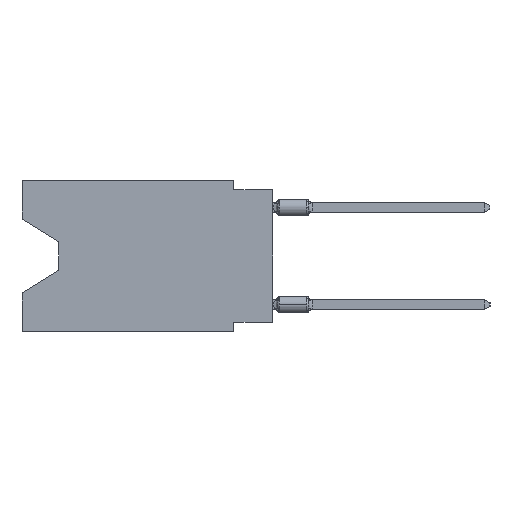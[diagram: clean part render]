
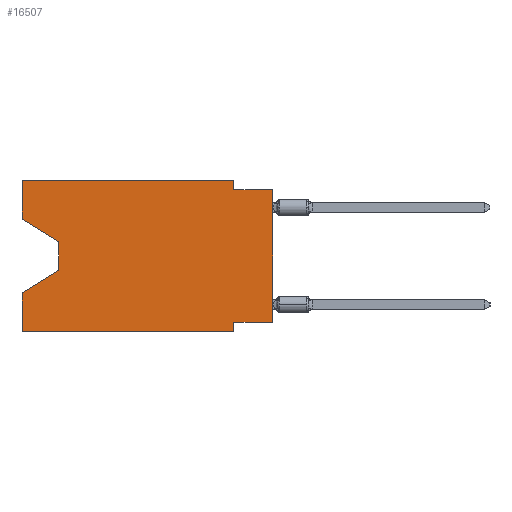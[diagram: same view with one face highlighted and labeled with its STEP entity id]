
A CAD part, left-side view. The second image highlights one B-rep face of the part: STEP entity #16507.
In plain terms, the highlighted planar face has unit normal (-1, 0, 0).
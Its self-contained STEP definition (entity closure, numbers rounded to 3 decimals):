
#143 = EDGE_CURVE ( 'NONE', #8141, #33290, #33464, .T. ) ;
#240 = CARTESIAN_POINT ( 'NONE',  ( 0., 16.383, 0. ) ) ;
#406 = ORIENTED_EDGE ( 'NONE', *, *, #2234, .F. ) ;
#1386 = DIRECTION ( 'NONE',  ( 0., 0.855, -0.519 ) ) ;
#1780 = EDGE_CURVE ( 'NONE', #19419, #35402, #20577, .T. ) ;
#2004 = CARTESIAN_POINT ( 'NONE',  ( 0., 16.383, 0. ) ) ;
#2234 = EDGE_CURVE ( 'NONE', #33290, #3593, #14030, .T. ) ;
#2667 = EDGE_CURVE ( 'NONE', #3593, #3488, #34184, .T. ) ;
#2804 = EDGE_CURVE ( 'NONE', #35402, #36213, #29673, .T. ) ;
#3255 = CARTESIAN_POINT ( 'NONE',  ( 0., 16.383, -9.906 ) ) ;
#3257 = ORIENTED_EDGE ( 'NONE', *, *, #29167, .T. ) ;
#3488 = VERTEX_POINT ( 'NONE', #28493 ) ;
#3593 = VERTEX_POINT ( 'NONE', #12446 ) ;
#3602 = DIRECTION ( 'NONE',  ( 1., 0., 0. ) ) ;
#4356 = VECTOR ( 'NONE', #14814, 1000. ) ;
#5134 = FACE_OUTER_BOUND ( 'NONE', #15252, .T. ) ;
#5652 = EDGE_CURVE ( 'NONE', #23869, #19419, #35515, .T. ) ;
#6834 = CARTESIAN_POINT ( 'NONE',  ( 0., 16.383, -2.546 ) ) ;
#7068 = CARTESIAN_POINT ( 'NONE',  ( 0., 0., 0. ) ) ;
#8136 = VECTOR ( 'NONE', #14589, 1000. ) ;
#8141 = VERTEX_POINT ( 'NONE', #2004 ) ;
#8772 = CARTESIAN_POINT ( 'NONE',  ( 0., 13.97, -5.893 ) ) ;
#9000 = DIRECTION ( 'NONE',  ( 0., 1., 0. ) ) ;
#9156 = CARTESIAN_POINT ( 'NONE',  ( 0., 16.383, -9.906 ) ) ;
#9291 = VECTOR ( 'NONE', #33102, 1000. ) ;
#9970 = VECTOR ( 'NONE', #23362, 1000. ) ;
#10121 = EDGE_CURVE ( 'NONE', #25347, #3488, #35561, .T. ) ;
#10722 = ORIENTED_EDGE ( 'NONE', *, *, #14795, .F. ) ;
#11436 = CARTESIAN_POINT ( 'NONE',  ( 0., 16.383, -2.546 ) ) ;
#11579 = DIRECTION ( 'NONE',  ( 0., 0., 1. ) ) ;
#11850 = CARTESIAN_POINT ( 'NONE',  ( 0., 16.383, 0. ) ) ;
#11993 = CARTESIAN_POINT ( 'NONE',  ( 0., 13.97, -4.013 ) ) ;
#12225 = VECTOR ( 'NONE', #26142, 1000. ) ;
#12284 = CARTESIAN_POINT ( 'NONE',  ( 0., 16.383, -7.36 ) ) ;
#12446 = CARTESIAN_POINT ( 'NONE',  ( 0., 2.54, -0.635 ) ) ;
#13673 = PLANE ( 'NONE',  #35334 ) ;
#14030 = LINE ( 'NONE', #19797, #24277 ) ;
#14190 = VERTEX_POINT ( 'NONE', #9156 ) ;
#14589 = DIRECTION ( 'NONE',  ( 0., -1., 0. ) ) ;
#14795 = EDGE_CURVE ( 'NONE', #25347, #17479, #17368, .T. ) ;
#14814 = DIRECTION ( 'NONE',  ( 0., 0., 1. ) ) ;
#15243 = ORIENTED_EDGE ( 'NONE', *, *, #2804, .T. ) ;
#15252 = EDGE_LOOP ( 'NONE', ( #28697, #23239, #15243, #21667, #3257, #30619, #10722, #22334, #18786, #406, #24752, #32365 ) ) ;
#15467 = LINE ( 'NONE', #23489, #28658 ) ;
#15863 = CARTESIAN_POINT ( 'NONE',  ( 0., 0., -9.271 ) ) ;
#16212 = VECTOR ( 'NONE', #9000, 1000. ) ;
#16491 = CARTESIAN_POINT ( 'NONE',  ( 0., 2.54, 0. ) ) ;
#16507 = ADVANCED_FACE ( 'NONE', ( #5134 ), #13673, .F. ) ;
#16673 = VECTOR ( 'NONE', #18403, 1000. ) ;
#17368 = LINE ( 'NONE', #35244, #16212 ) ;
#17479 = VERTEX_POINT ( 'NONE', #35667 ) ;
#17580 = CARTESIAN_POINT ( 'NONE',  ( 0., 0., -0.635 ) ) ;
#18403 = DIRECTION ( 'NONE',  ( 0., 0., 1. ) ) ;
#18786 = ORIENTED_EDGE ( 'NONE', *, *, #2667, .F. ) ;
#19098 = VERTEX_POINT ( 'NONE', #22338 ) ;
#19419 = VERTEX_POINT ( 'NONE', #21321 ) ;
#19797 = CARTESIAN_POINT ( 'NONE',  ( 0., 2.54, 0. ) ) ;
#20577 = LINE ( 'NONE', #11993, #9970 ) ;
#20902 = LINE ( 'NONE', #3255, #8136 ) ;
#21321 = CARTESIAN_POINT ( 'NONE',  ( 0., 13.97, -4.013 ) ) ;
#21667 = ORIENTED_EDGE ( 'NONE', *, *, #33805, .F. ) ;
#22334 = ORIENTED_EDGE ( 'NONE', *, *, #10121, .T. ) ;
#22338 = CARTESIAN_POINT ( 'NONE',  ( 0., 2.54, -9.906 ) ) ;
#23239 = ORIENTED_EDGE ( 'NONE', *, *, #1780, .T. ) ;
#23362 = DIRECTION ( 'NONE',  ( 0., 0., -1. ) ) ;
#23489 = CARTESIAN_POINT ( 'NONE',  ( 0., 2.54, -9.906 ) ) ;
#23869 = VERTEX_POINT ( 'NONE', #11436 ) ;
#23957 = EDGE_CURVE ( 'NONE', #17479, #19098, #15467, .T. ) ;
#24277 = VECTOR ( 'NONE', #36766, 1000. ) ;
#24752 = ORIENTED_EDGE ( 'NONE', *, *, #143, .F. ) ;
#24812 = VECTOR ( 'NONE', #32722, 1000. ) ;
#25347 = VERTEX_POINT ( 'NONE', #15863 ) ;
#26142 = DIRECTION ( 'NONE',  ( 0., -1., 0. ) ) ;
#28493 = CARTESIAN_POINT ( 'NONE',  ( 0., 0., -0.635 ) ) ;
#28526 = LINE ( 'NONE', #240, #35306 ) ;
#28658 = VECTOR ( 'NONE', #29630, 1000. ) ;
#28697 = ORIENTED_EDGE ( 'NONE', *, *, #5652, .T. ) ;
#29167 = EDGE_CURVE ( 'NONE', #14190, #19098, #20902, .T. ) ;
#29630 = DIRECTION ( 'NONE',  ( 0., 0., -1. ) ) ;
#29673 = LINE ( 'NONE', #32293, #33658 ) ;
#30619 = ORIENTED_EDGE ( 'NONE', *, *, #23957, .F. ) ;
#32293 = CARTESIAN_POINT ( 'NONE',  ( 0., 13.97, -5.893 ) ) ;
#32365 = ORIENTED_EDGE ( 'NONE', *, *, #33077, .F. ) ;
#32722 = DIRECTION ( 'NONE',  ( 0., -0.855, -0.519 ) ) ;
#33077 = EDGE_CURVE ( 'NONE', #23869, #8141, #34770, .T. ) ;
#33102 = DIRECTION ( 'NONE',  ( 0., -1., 0. ) ) ;
#33290 = VERTEX_POINT ( 'NONE', #16491 ) ;
#33464 = LINE ( 'NONE', #36265, #9291 ) ;
#33658 = VECTOR ( 'NONE', #1386, 1000. ) ;
#33805 = EDGE_CURVE ( 'NONE', #14190, #36213, #28526, .T. ) ;
#34184 = LINE ( 'NONE', #17580, #12225 ) ;
#34700 = DIRECTION ( 'NONE',  ( 0., 0., -1. ) ) ;
#34770 = LINE ( 'NONE', #11850, #4356 ) ;
#34887 = CARTESIAN_POINT ( 'NONE',  ( 0., 16.383, 0. ) ) ;
#35244 = CARTESIAN_POINT ( 'NONE',  ( 0., 0., -9.271 ) ) ;
#35306 = VECTOR ( 'NONE', #11579, 1000. ) ;
#35334 = AXIS2_PLACEMENT_3D ( 'NONE', #34887, #3602, #34700 ) ;
#35402 = VERTEX_POINT ( 'NONE', #8772 ) ;
#35515 = LINE ( 'NONE', #6834, #24812 ) ;
#35561 = LINE ( 'NONE', #7068, #16673 ) ;
#35667 = CARTESIAN_POINT ( 'NONE',  ( 0., 2.54, -9.271 ) ) ;
#36213 = VERTEX_POINT ( 'NONE', #12284 ) ;
#36265 = CARTESIAN_POINT ( 'NONE',  ( 0., 16.383, 0. ) ) ;
#36766 = DIRECTION ( 'NONE',  ( 0., 0., -1. ) ) ;
